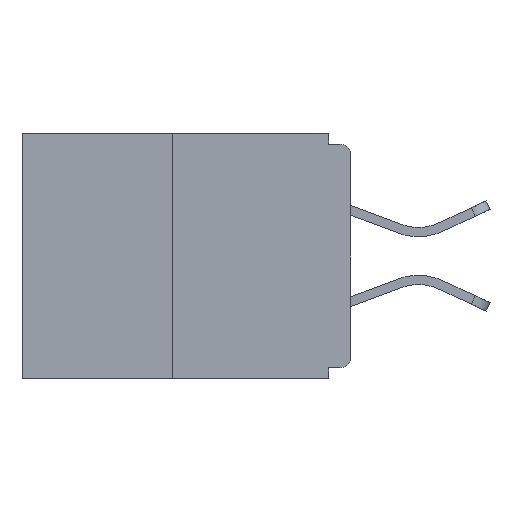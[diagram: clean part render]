
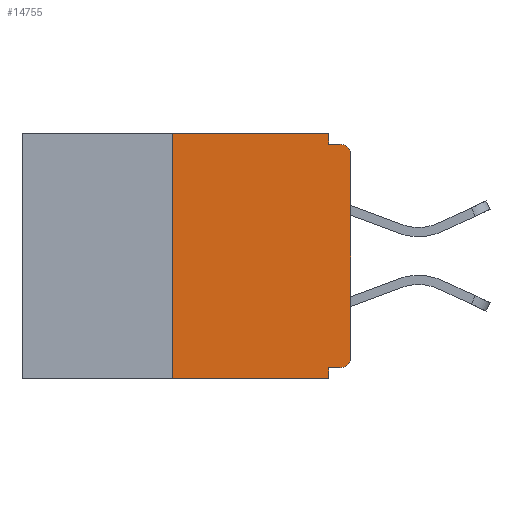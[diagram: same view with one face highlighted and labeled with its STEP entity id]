
A CAD part, left-side view. The second image highlights one B-rep face of the part: STEP entity #14755.
In plain terms, the highlighted planar face has unit normal (-1, 0, 0).
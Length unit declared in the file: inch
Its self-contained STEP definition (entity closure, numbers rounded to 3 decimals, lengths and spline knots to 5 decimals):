
#559 = ORIENTED_EDGE ( 'NONE', *, *, #5777, .F. ) ;
#676 = EDGE_CURVE ( 'NONE', #31112, #23722, #25686, .T. ) ;
#831 = VECTOR ( 'NONE', #8195, 39.37008 ) ;
#844 = DIRECTION ( 'NONE',  ( 0., 1., 0. ) ) ;
#1243 = DIRECTION ( 'NONE',  ( 0., 0., -1. ) ) ;
#1763 = ORIENTED_EDGE ( 'NONE', *, *, #29068, .F. ) ;
#2440 = AXIS2_PLACEMENT_3D ( 'NONE', #21021, #28314, #6314 ) ;
#3047 = EDGE_CURVE ( 'NONE', #7047, #31369, #25946, .T. ) ;
#3315 = CARTESIAN_POINT ( 'NONE',  ( 0., 0.031, -0.343 ) ) ;
#3380 = VERTEX_POINT ( 'NONE', #21222 ) ;
#4198 = EDGE_CURVE ( 'NONE', #11203, #11043, #15666, .T. ) ;
#4210 = CARTESIAN_POINT ( 'NONE',  ( 0., 0.031, -0.015 ) ) ;
#4547 = ORIENTED_EDGE ( 'NONE', *, *, #11982, .T. ) ;
#5595 = CARTESIAN_POINT ( 'NONE',  ( 0., 0.25, 0. ) ) ;
#5704 = VERTEX_POINT ( 'NONE', #20262 ) ;
#5777 = EDGE_CURVE ( 'NONE', #27993, #11203, #9465, .T. ) ;
#6314 = DIRECTION ( 'NONE',  ( 0., 0., -1. ) ) ;
#6509 = DIRECTION ( 'NONE',  ( 0., 0., -1. ) ) ;
#7047 = VERTEX_POINT ( 'NONE', #15446 ) ;
#7328 = ORIENTED_EDGE ( 'NONE', *, *, #20017, .F. ) ;
#8030 = ORIENTED_EDGE ( 'NONE', *, *, #676, .T. ) ;
#8195 = DIRECTION ( 'NONE',  ( 0., 0., -1. ) ) ;
#8274 = CARTESIAN_POINT ( 'NONE',  ( 0., 0., -0.328 ) ) ;
#9324 = ORIENTED_EDGE ( 'NONE', *, *, #13479, .T. ) ;
#9465 = LINE ( 'NONE', #15605, #14817 ) ;
#11043 = VERTEX_POINT ( 'NONE', #12991 ) ;
#11203 = VERTEX_POINT ( 'NONE', #4210 ) ;
#11224 = EDGE_CURVE ( 'NONE', #3380, #11043, #14968, .T. ) ;
#11463 = PLANE ( 'NONE',  #2440 ) ;
#11982 = EDGE_CURVE ( 'NONE', #23722, #3380, #25565, .T. ) ;
#12830 = AXIS2_PLACEMENT_3D ( 'NONE', #25356, #22923, #1243 ) ;
#12991 = CARTESIAN_POINT ( 'NONE',  ( 0., 0.015, -0.015 ) ) ;
#13174 = LINE ( 'NONE', #5595, #26830 ) ;
#13222 = DIRECTION ( 'NONE',  ( 0., 0., 1. ) ) ;
#13479 = EDGE_CURVE ( 'NONE', #16834, #31369, #22797, .T. ) ;
#13731 = LINE ( 'NONE', #8274, #30800 ) ;
#13773 = DIRECTION ( 'NONE',  ( 0., -1., 0. ) ) ;
#14512 = DIRECTION ( 'NONE',  ( 0., 0., 1. ) ) ;
#14755 = ADVANCED_FACE ( 'NONE', ( #29225 ), #11463, .F. ) ;
#14817 = VECTOR ( 'NONE', #20473, 39.37008 ) ;
#14844 = ORIENTED_EDGE ( 'NONE', *, *, #3047, .F. ) ;
#14968 = CIRCLE ( 'NONE', #18905, 0.015 ) ;
#15224 = CARTESIAN_POINT ( 'NONE',  ( 0., 0.015, -0.03 ) ) ;
#15446 = CARTESIAN_POINT ( 'NONE',  ( 0., 0.031, -0.328 ) ) ;
#15605 = CARTESIAN_POINT ( 'NONE',  ( 0., 0.031, 0. ) ) ;
#15666 = LINE ( 'NONE', #18836, #23244 ) ;
#16607 = VECTOR ( 'NONE', #13773, 39.37008 ) ;
#16834 = VERTEX_POINT ( 'NONE', #25002 ) ;
#18836 = CARTESIAN_POINT ( 'NONE',  ( 0., 0., -0.015 ) ) ;
#18905 = AXIS2_PLACEMENT_3D ( 'NONE', #15224, #21335, #6509 ) ;
#19097 = DIRECTION ( 'NONE',  ( 0., -1., 0. ) ) ;
#19137 = VECTOR ( 'NONE', #14512, 39.37008 ) ;
#20017 = EDGE_CURVE ( 'NONE', #31112, #7047, #13731, .T. ) ;
#20262 = CARTESIAN_POINT ( 'NONE',  ( 0., 0.25, 0. ) ) ;
#20473 = DIRECTION ( 'NONE',  ( 0., 0., -1. ) ) ;
#21021 = CARTESIAN_POINT ( 'NONE',  ( 0., 0.46, 0. ) ) ;
#21222 = CARTESIAN_POINT ( 'NONE',  ( 0., 0., -0.03 ) ) ;
#21335 = DIRECTION ( 'NONE',  ( -1., 0., 0. ) ) ;
#21423 = CARTESIAN_POINT ( 'NONE',  ( 0., 0.46, -0.343 ) ) ;
#22600 = CARTESIAN_POINT ( 'NONE',  ( 0., 0.031, -0.343 ) ) ;
#22797 = LINE ( 'NONE', #21423, #25074 ) ;
#22923 = DIRECTION ( 'NONE',  ( -1., 0., 0. ) ) ;
#23244 = VECTOR ( 'NONE', #28428, 39.37008 ) ;
#23722 = VERTEX_POINT ( 'NONE', #25987 ) ;
#24143 = CARTESIAN_POINT ( 'NONE',  ( 0., 0., 0. ) ) ;
#25002 = CARTESIAN_POINT ( 'NONE',  ( 0., 0.25, -0.343 ) ) ;
#25074 = VECTOR ( 'NONE', #19097, 39.37008 ) ;
#25356 = CARTESIAN_POINT ( 'NONE',  ( 0., 0.015, -0.313 ) ) ;
#25446 = ORIENTED_EDGE ( 'NONE', *, *, #11224, .T. ) ;
#25565 = LINE ( 'NONE', #24143, #19137 ) ;
#25686 = CIRCLE ( 'NONE', #12830, 0.015 ) ;
#25946 = LINE ( 'NONE', #3315, #831 ) ;
#25987 = CARTESIAN_POINT ( 'NONE',  ( 0., 0., -0.313 ) ) ;
#26390 = EDGE_LOOP ( 'NONE', ( #1763, #28513, #9324, #14844, #7328, #8030, #4547, #25446, #28480, #559 ) ) ;
#26830 = VECTOR ( 'NONE', #13222, 39.37008 ) ;
#27532 = LINE ( 'NONE', #28266, #16607 ) ;
#27966 = CARTESIAN_POINT ( 'NONE',  ( 0., 0.031, 0. ) ) ;
#27993 = VERTEX_POINT ( 'NONE', #27966 ) ;
#28266 = CARTESIAN_POINT ( 'NONE',  ( 0., 0.46, 0. ) ) ;
#28314 = DIRECTION ( 'NONE',  ( 1., 0., 0. ) ) ;
#28428 = DIRECTION ( 'NONE',  ( 0., -1., 0. ) ) ;
#28471 = CARTESIAN_POINT ( 'NONE',  ( 0., 0.015, -0.328 ) ) ;
#28480 = ORIENTED_EDGE ( 'NONE', *, *, #4198, .F. ) ;
#28513 = ORIENTED_EDGE ( 'NONE', *, *, #28881, .F. ) ;
#28881 = EDGE_CURVE ( 'NONE', #16834, #5704, #13174, .T. ) ;
#29068 = EDGE_CURVE ( 'NONE', #5704, #27993, #27532, .T. ) ;
#29225 = FACE_OUTER_BOUND ( 'NONE', #26390, .T. ) ;
#30800 = VECTOR ( 'NONE', #844, 39.37008 ) ;
#31112 = VERTEX_POINT ( 'NONE', #28471 ) ;
#31369 = VERTEX_POINT ( 'NONE', #22600 ) ;
